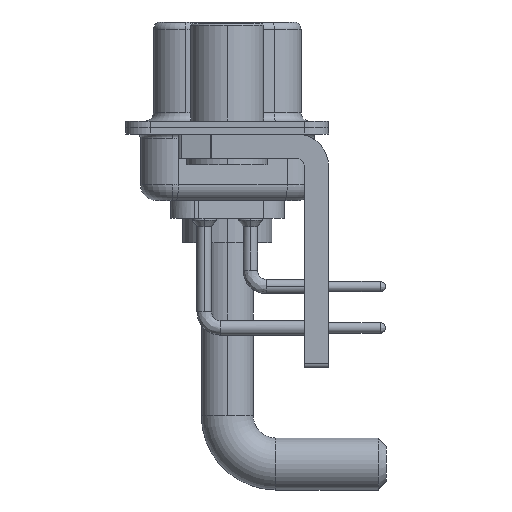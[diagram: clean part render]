
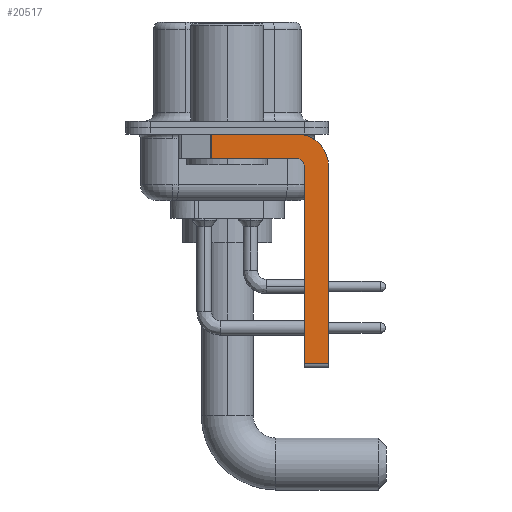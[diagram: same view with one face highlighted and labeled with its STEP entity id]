
A CAD part, left-side view. The second image highlights one B-rep face of the part: STEP entity #20517.
In plain terms, the highlighted planar face has unit normal (-1, 0, 0).
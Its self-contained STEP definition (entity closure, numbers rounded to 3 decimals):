
#367 = CIRCLE ( 'NONE', #10960, 0.5 ) ;
#849 = CARTESIAN_POINT ( 'NONE',  ( -2.9, -4.25, -1.9 ) ) ;
#1353 = LINE ( 'NONE', #27623, #13770 ) ;
#1398 = FACE_OUTER_BOUND ( 'NONE', #26587, .T. ) ;
#1656 = LINE ( 'NONE', #21197, #8969 ) ;
#2104 = LINE ( 'NONE', #8317, #19132 ) ;
#2321 = ORIENTED_EDGE ( 'NONE', *, *, #27549, .F. ) ;
#2604 = CIRCLE ( 'NONE', #9513, 2. ) ;
#3066 = LINE ( 'NONE', #7408, #3830 ) ;
#3550 = CARTESIAN_POINT ( 'NONE',  ( -2.9, -4.25, -0.4 ) ) ;
#3830 = VECTOR ( 'NONE', #11842, 1000. ) ;
#3987 = DIRECTION ( 'NONE',  ( 0., 0., -1. ) ) ;
#4414 = CARTESIAN_POINT ( 'NONE',  ( -2.9, 0.978, -1.9 ) ) ;
#4591 = DIRECTION ( 'NONE',  ( 1., 0., 0. ) ) ;
#5796 = CARTESIAN_POINT ( 'NONE',  ( -2.9, -4.25, -1.9 ) ) ;
#6052 = CARTESIAN_POINT ( 'NONE',  ( -2.9, 0.978, -1.9 ) ) ;
#6460 = CARTESIAN_POINT ( 'NONE',  ( -2.9, -4.25, -2.4 ) ) ;
#6901 = CARTESIAN_POINT ( 'NONE',  ( -2.9, -6.25, -14.55 ) ) ;
#7408 = CARTESIAN_POINT ( 'NONE',  ( -2.9, -4.75, -14.8 ) ) ;
#7522 = EDGE_CURVE ( 'NONE', #8487, #11494, #20539, .T. ) ;
#7662 = VECTOR ( 'NONE', #3987, 1000. ) ;
#7983 = DIRECTION ( 'NONE',  ( 0., -1., 0. ) ) ;
#8317 = CARTESIAN_POINT ( 'NONE',  ( -2.9, -6.25, -2.4 ) ) ;
#8487 = VERTEX_POINT ( 'NONE', #5796 ) ;
#8635 = CARTESIAN_POINT ( 'NONE',  ( -2.9, -4.25, -2.4 ) ) ;
#8969 = VECTOR ( 'NONE', #10448, 1000. ) ;
#9397 = VERTEX_POINT ( 'NONE', #13602 ) ;
#9513 = AXIS2_PLACEMENT_3D ( 'NONE', #6460, #4591, #19822 ) ;
#9924 = ORIENTED_EDGE ( 'NONE', *, *, #20282, .F. ) ;
#10110 = CARTESIAN_POINT ( 'NONE',  ( -2.9, -6.25, -2.4 ) ) ;
#10181 = DIRECTION ( 'NONE',  ( 0., 0., -1. ) ) ;
#10448 = DIRECTION ( 'NONE',  ( 0., -1., 0. ) ) ;
#10960 = AXIS2_PLACEMENT_3D ( 'NONE', #8635, #15378, #25827 ) ;
#10988 = EDGE_CURVE ( 'NONE', #23134, #21946, #1353, .T. ) ;
#10991 = ORIENTED_EDGE ( 'NONE', *, *, #15926, .T. ) ;
#11494 = VERTEX_POINT ( 'NONE', #6052 ) ;
#11775 = VECTOR ( 'NONE', #27120, 1000. ) ;
#11842 = DIRECTION ( 'NONE',  ( 0., 0., 1. ) ) ;
#11883 = ORIENTED_EDGE ( 'NONE', *, *, #10988, .F. ) ;
#12170 = CARTESIAN_POINT ( 'NONE',  ( -2.9, -4.25, -2.4 ) ) ;
#12609 = DIRECTION ( 'NONE',  ( 0., 0., -1. ) ) ;
#13602 = CARTESIAN_POINT ( 'NONE',  ( -2.9, -4.75, -14.55 ) ) ;
#13770 = VECTOR ( 'NONE', #7983, 1000. ) ;
#14486 = ORIENTED_EDGE ( 'NONE', *, *, #27835, .T. ) ;
#14882 = ORIENTED_EDGE ( 'NONE', *, *, #27775, .F. ) ;
#15378 = DIRECTION ( 'NONE',  ( -1., 0., 0. ) ) ;
#15926 = EDGE_CURVE ( 'NONE', #9397, #23025, #1656, .T. ) ;
#16050 = VERTEX_POINT ( 'NONE', #19772 ) ;
#16237 = EDGE_CURVE ( 'NONE', #9397, #16050, #3066, .T. ) ;
#16363 = DIRECTION ( 'NONE',  ( 1., 0., 0. ) ) ;
#19132 = VECTOR ( 'NONE', #12609, 1000. ) ;
#19772 = CARTESIAN_POINT ( 'NONE',  ( -2.9, -4.75, -2.4 ) ) ;
#19795 = ORIENTED_EDGE ( 'NONE', *, *, #16237, .F. ) ;
#19822 = DIRECTION ( 'NONE',  ( 0., 0., -1. ) ) ;
#20282 = EDGE_CURVE ( 'NONE', #16050, #8487, #367, .T. ) ;
#20517 = ADVANCED_FACE ( 'NONE', ( #1398 ), #27804, .F. ) ;
#20539 = LINE ( 'NONE', #849, #11775 ) ;
#20760 = ORIENTED_EDGE ( 'NONE', *, *, #7522, .F. ) ;
#21108 = VERTEX_POINT ( 'NONE', #10110 ) ;
#21197 = CARTESIAN_POINT ( 'NONE',  ( -2.9, -4.25, -14.55 ) ) ;
#21946 = VERTEX_POINT ( 'NONE', #3550 ) ;
#23025 = VERTEX_POINT ( 'NONE', #6901 ) ;
#23134 = VERTEX_POINT ( 'NONE', #26688 ) ;
#23537 = AXIS2_PLACEMENT_3D ( 'NONE', #12170, #16363, #10181 ) ;
#25659 = LINE ( 'NONE', #4414, #7662 ) ;
#25827 = DIRECTION ( 'NONE',  ( 0., 0., 1. ) ) ;
#26587 = EDGE_LOOP ( 'NONE', ( #11883, #14486, #20760, #9924, #19795, #10991, #14882, #2321 ) ) ;
#26688 = CARTESIAN_POINT ( 'NONE',  ( -2.9, 0.978, -0.4 ) ) ;
#27120 = DIRECTION ( 'NONE',  ( 0., 1., 0. ) ) ;
#27549 = EDGE_CURVE ( 'NONE', #21946, #21108, #2604, .T. ) ;
#27623 = CARTESIAN_POINT ( 'NONE',  ( -2.9, 3., -0.4 ) ) ;
#27775 = EDGE_CURVE ( 'NONE', #21108, #23025, #2104, .T. ) ;
#27804 = PLANE ( 'NONE',  #23537 ) ;
#27835 = EDGE_CURVE ( 'NONE', #23134, #11494, #25659, .T. ) ;
